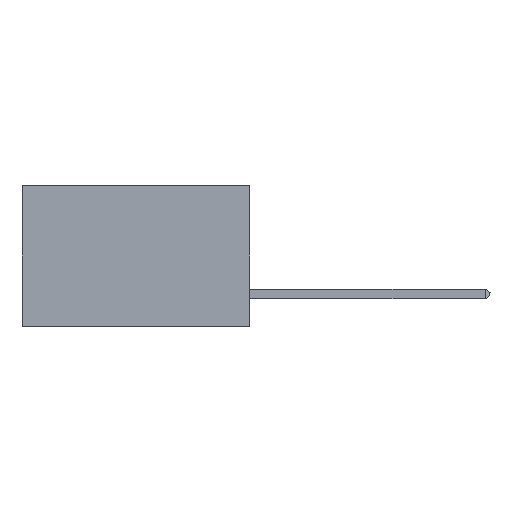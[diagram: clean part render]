
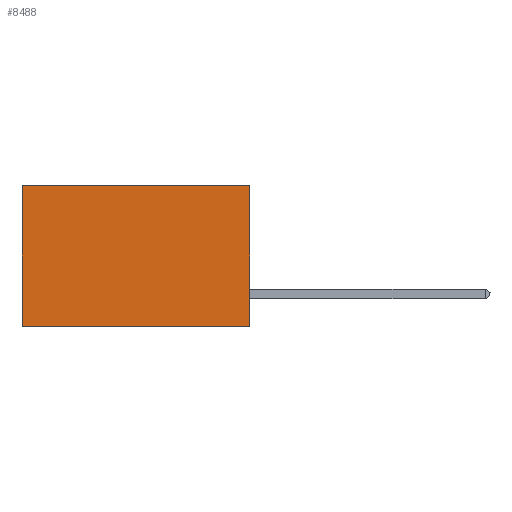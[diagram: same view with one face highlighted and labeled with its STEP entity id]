
A CAD part, left-side view. The second image highlights one B-rep face of the part: STEP entity #8488.
In plain terms, the highlighted planar face has unit normal (-1, 0, 0).
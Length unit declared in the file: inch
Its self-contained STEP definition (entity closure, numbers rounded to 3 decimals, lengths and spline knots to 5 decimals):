
#1813 = EDGE_LOOP ( 'NONE', ( #45335, #3789, #14522, #6953 ) ) ;
#1982 = DIRECTION ( 'NONE',  ( 0., 0., -1. ) ) ;
#3695 = VECTOR ( 'NONE', #1982, 39.37008 ) ;
#3716 = DIRECTION ( 'NONE',  ( 0., 0., -1. ) ) ;
#3789 = ORIENTED_EDGE ( 'NONE', *, *, #10963, .F. ) ;
#6036 = CARTESIAN_POINT ( 'NONE',  ( 0.2875, 0., 0. ) ) ;
#6302 = LINE ( 'NONE', #14629, #35127 ) ;
#6953 = ORIENTED_EDGE ( 'NONE', *, *, #40991, .T. ) ;
#7272 = VERTEX_POINT ( 'NONE', #41833 ) ;
#7288 = LINE ( 'NONE', #6036, #3695 ) ;
#7674 = VECTOR ( 'NONE', #38496, 39.37008 ) ;
#8324 = EDGE_CURVE ( 'NONE', #31595, #43833, #7288, .T. ) ;
#8488 = ADVANCED_FACE ( 'NONE', ( #15104 ), #45411, .F. ) ;
#9408 = CARTESIAN_POINT ( 'NONE',  ( 0.2875, 0., 0. ) ) ;
#10186 = CARTESIAN_POINT ( 'NONE',  ( 0.2875, 0.6, 0. ) ) ;
#10963 = EDGE_CURVE ( 'NONE', #43833, #7272, #25756, .T. ) ;
#12046 = VERTEX_POINT ( 'NONE', #10186 ) ;
#14002 = AXIS2_PLACEMENT_3D ( 'NONE', #22551, #40005, #3716 ) ;
#14522 = ORIENTED_EDGE ( 'NONE', *, *, #8324, .F. ) ;
#14629 = CARTESIAN_POINT ( 'NONE',  ( 0.2875, 0., 0. ) ) ;
#15104 = FACE_OUTER_BOUND ( 'NONE', #1813, .T. ) ;
#15481 = EDGE_CURVE ( 'NONE', #12046, #7272, #27256, .T. ) ;
#16931 = VECTOR ( 'NONE', #32631, 39.37008 ) ;
#20716 = CARTESIAN_POINT ( 'NONE',  ( 0.2875, 0., -0.37 ) ) ;
#22551 = CARTESIAN_POINT ( 'NONE',  ( 0.2875, 0., 0. ) ) ;
#25756 = LINE ( 'NONE', #48441, #7674 ) ;
#27256 = LINE ( 'NONE', #48315, #16931 ) ;
#31595 = VERTEX_POINT ( 'NONE', #9408 ) ;
#32631 = DIRECTION ( 'NONE',  ( 0., 0., -1. ) ) ;
#35127 = VECTOR ( 'NONE', #45599, 39.37008 ) ;
#38496 = DIRECTION ( 'NONE',  ( 0., 1., 0. ) ) ;
#40005 = DIRECTION ( 'NONE',  ( 1., 0., 0. ) ) ;
#40991 = EDGE_CURVE ( 'NONE', #31595, #12046, #6302, .T. ) ;
#41833 = CARTESIAN_POINT ( 'NONE',  ( 0.2875, 0.6, -0.37 ) ) ;
#43833 = VERTEX_POINT ( 'NONE', #20716 ) ;
#45335 = ORIENTED_EDGE ( 'NONE', *, *, #15481, .T. ) ;
#45411 = PLANE ( 'NONE',  #14002 ) ;
#45599 = DIRECTION ( 'NONE',  ( 0., 1., 0. ) ) ;
#48315 = CARTESIAN_POINT ( 'NONE',  ( 0.2875, 0.6, 0. ) ) ;
#48441 = CARTESIAN_POINT ( 'NONE',  ( 0.2875, 0., -0.37 ) ) ;
